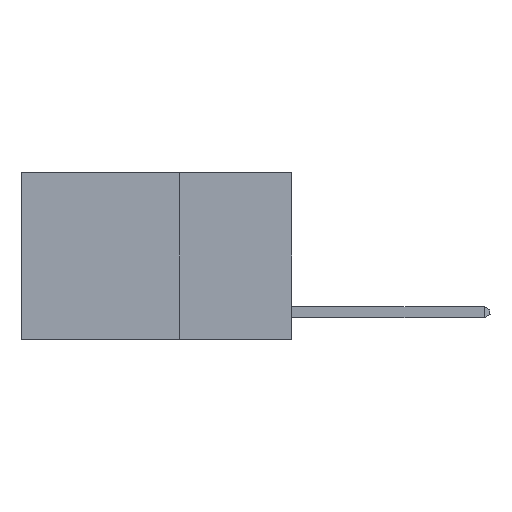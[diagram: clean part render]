
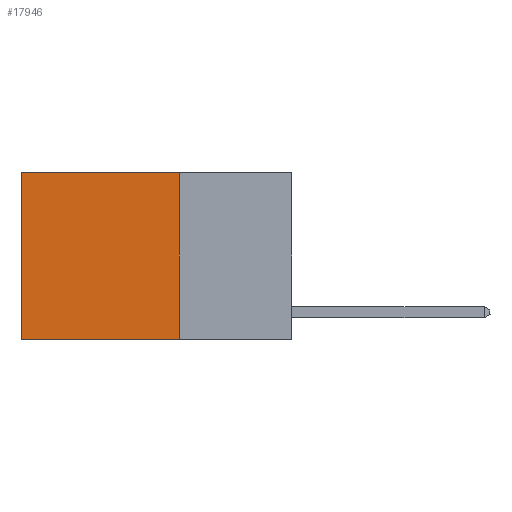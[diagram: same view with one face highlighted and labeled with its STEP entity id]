
A CAD part, left-side view. The second image highlights one B-rep face of the part: STEP entity #17946.
In plain terms, the highlighted planar face has unit normal (-1, 0, 0).
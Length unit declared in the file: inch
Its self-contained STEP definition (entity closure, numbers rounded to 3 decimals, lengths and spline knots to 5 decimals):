
#1170 = CARTESIAN_POINT ( 'NONE',  ( 0.2625, 0.25, 0. ) ) ;
#1440 = LINE ( 'NONE', #1170, #26165 ) ;
#1584 = VECTOR ( 'NONE', #16133, 39.37008 ) ;
#1732 = EDGE_LOOP ( 'NONE', ( #22995, #2809, #12845, #12319 ) ) ;
#2809 = ORIENTED_EDGE ( 'NONE', *, *, #13524, .F. ) ;
#2878 = AXIS2_PLACEMENT_3D ( 'NONE', #3988, #14179, #22348 ) ;
#3075 = LINE ( 'NONE', #6692, #26503 ) ;
#3988 = CARTESIAN_POINT ( 'NONE',  ( 0.2625, 0.25, 0. ) ) ;
#4074 = EDGE_CURVE ( 'NONE', #17293, #13238, #3075, .T. ) ;
#6007 = PLANE ( 'NONE',  #2878 ) ;
#6692 = CARTESIAN_POINT ( 'NONE',  ( 0.2625, 0.25, 0. ) ) ;
#6950 = EDGE_CURVE ( 'NONE', #24585, #18097, #12256, .T. ) ;
#10008 = LINE ( 'NONE', #22039, #13461 ) ;
#10828 = CARTESIAN_POINT ( 'NONE',  ( 0.2625, 0.25, -0.37 ) ) ;
#12256 = LINE ( 'NONE', #12524, #1584 ) ;
#12319 = ORIENTED_EDGE ( 'NONE', *, *, #21730, .T. ) ;
#12524 = CARTESIAN_POINT ( 'NONE',  ( 0.2625, 0.6, 0. ) ) ;
#12845 = ORIENTED_EDGE ( 'NONE', *, *, #4074, .F. ) ;
#13238 = VERTEX_POINT ( 'NONE', #10828 ) ;
#13461 = VECTOR ( 'NONE', #18424, 39.37008 ) ;
#13524 = EDGE_CURVE ( 'NONE', #13238, #18097, #10008, .T. ) ;
#14179 = DIRECTION ( 'NONE',  ( 1., 0., 0. ) ) ;
#15813 = CARTESIAN_POINT ( 'NONE',  ( 0.2625, 0.25, 0. ) ) ;
#16133 = DIRECTION ( 'NONE',  ( 0., 0., -1. ) ) ;
#17293 = VERTEX_POINT ( 'NONE', #15813 ) ;
#17499 = DIRECTION ( 'NONE',  ( 0., 1., 0. ) ) ;
#17946 = ADVANCED_FACE ( 'NONE', ( #24370 ), #6007, .F. ) ;
#18097 = VERTEX_POINT ( 'NONE', #19497 ) ;
#18424 = DIRECTION ( 'NONE',  ( 0., 1., 0. ) ) ;
#19417 = DIRECTION ( 'NONE',  ( 0., 0., -1. ) ) ;
#19497 = CARTESIAN_POINT ( 'NONE',  ( 0.2625, 0.6, -0.37 ) ) ;
#19630 = CARTESIAN_POINT ( 'NONE',  ( 0.2625, 0.6, 0. ) ) ;
#21730 = EDGE_CURVE ( 'NONE', #17293, #24585, #1440, .T. ) ;
#22039 = CARTESIAN_POINT ( 'NONE',  ( 0.2625, 0.25, -0.37 ) ) ;
#22348 = DIRECTION ( 'NONE',  ( 0., 0., -1. ) ) ;
#22995 = ORIENTED_EDGE ( 'NONE', *, *, #6950, .T. ) ;
#24370 = FACE_OUTER_BOUND ( 'NONE', #1732, .T. ) ;
#24585 = VERTEX_POINT ( 'NONE', #19630 ) ;
#26165 = VECTOR ( 'NONE', #17499, 39.37008 ) ;
#26503 = VECTOR ( 'NONE', #19417, 39.37008 ) ;
